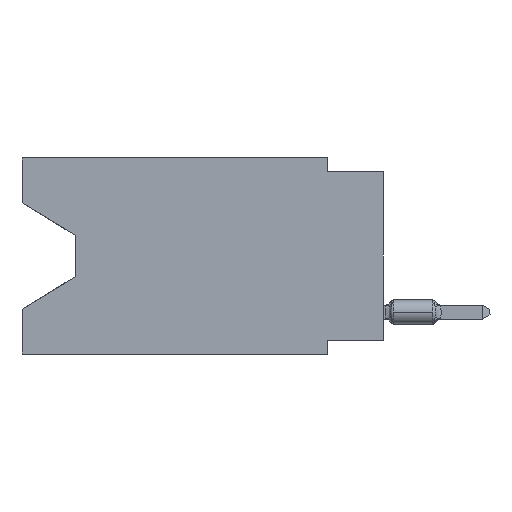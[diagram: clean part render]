
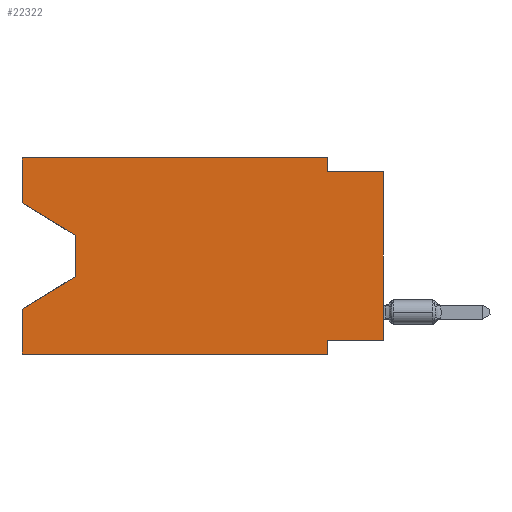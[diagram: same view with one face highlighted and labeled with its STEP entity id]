
A CAD part, left-side view. The second image highlights one B-rep face of the part: STEP entity #22322.
In plain terms, the highlighted planar face has unit normal (-1, 0, 0).
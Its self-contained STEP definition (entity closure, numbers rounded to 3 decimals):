
#72 = CARTESIAN_POINT ( 'NONE',  ( 0., 13.97, -3.505 ) ) ;
#204 = CARTESIAN_POINT ( 'NONE',  ( 0., 16.383, 0. ) ) ;
#387 = EDGE_CURVE ( 'NONE', #8166, #8063, #22553, .T. ) ;
#684 = EDGE_CURVE ( 'NONE', #5565, #3369, #23411, .T. ) ;
#905 = ORIENTED_EDGE ( 'NONE', *, *, #19188, .F. ) ;
#1069 = PLANE ( 'NONE',  #10532 ) ;
#1117 = DIRECTION ( 'NONE',  ( 0., -1., 0. ) ) ;
#1176 = ORIENTED_EDGE ( 'NONE', *, *, #18068, .F. ) ;
#1419 = ORIENTED_EDGE ( 'NONE', *, *, #15341, .T. ) ;
#1423 = VECTOR ( 'NONE', #16731, 1000. ) ;
#1515 = FACE_OUTER_BOUND ( 'NONE', #16196, .T. ) ;
#1603 = VECTOR ( 'NONE', #15028, 1000. ) ;
#1695 = CARTESIAN_POINT ( 'NONE',  ( 0., 16.383, -8.89 ) ) ;
#1734 = CARTESIAN_POINT ( 'NONE',  ( 0., 2.54, 0. ) ) ;
#1870 = ORIENTED_EDGE ( 'NONE', *, *, #10674, .F. ) ;
#1957 = VECTOR ( 'NONE', #16498, 1000. ) ;
#2122 = DIRECTION ( 'NONE',  ( 0., 0., -1. ) ) ;
#2438 = CARTESIAN_POINT ( 'NONE',  ( 0., 0., -0.635 ) ) ;
#2663 = CARTESIAN_POINT ( 'NONE',  ( 0., 16.383, 0. ) ) ;
#2787 = VERTEX_POINT ( 'NONE', #19200 ) ;
#3111 = EDGE_CURVE ( 'NONE', #17561, #3369, #4871, .T. ) ;
#3369 = VERTEX_POINT ( 'NONE', #23626 ) ;
#3672 = LINE ( 'NONE', #1734, #1957 ) ;
#4014 = DIRECTION ( 'NONE',  ( 0., 0., 1. ) ) ;
#4050 = ORIENTED_EDGE ( 'NONE', *, *, #8642, .T. ) ;
#4072 = LINE ( 'NONE', #204, #5555 ) ;
#4871 = LINE ( 'NONE', #19521, #14837 ) ;
#4877 = CARTESIAN_POINT ( 'NONE',  ( 0., 16.383, -8.89 ) ) ;
#4986 = VERTEX_POINT ( 'NONE', #11533 ) ;
#5273 = DIRECTION ( 'NONE',  ( 1., 0., 0. ) ) ;
#5416 = CARTESIAN_POINT ( 'NONE',  ( 0., 13.97, -5.385 ) ) ;
#5555 = VECTOR ( 'NONE', #23937, 1000. ) ;
#5565 = VERTEX_POINT ( 'NONE', #1695 ) ;
#5715 = CARTESIAN_POINT ( 'NONE',  ( 0., 16.383, 0. ) ) ;
#6098 = ORIENTED_EDGE ( 'NONE', *, *, #9938, .F. ) ;
#6109 = EDGE_CURVE ( 'NONE', #5565, #4986, #4072, .T. ) ;
#6717 = VERTEX_POINT ( 'NONE', #11790 ) ;
#6826 = ORIENTED_EDGE ( 'NONE', *, *, #3111, .F. ) ;
#7029 = LINE ( 'NONE', #16697, #22878 ) ;
#8004 = DIRECTION ( 'NONE',  ( 0., -1., 0. ) ) ;
#8063 = VERTEX_POINT ( 'NONE', #21836 ) ;
#8119 = LINE ( 'NONE', #2438, #21179 ) ;
#8166 = VERTEX_POINT ( 'NONE', #16743 ) ;
#8642 = EDGE_CURVE ( 'NONE', #2787, #6717, #15022, .T. ) ;
#8965 = ORIENTED_EDGE ( 'NONE', *, *, #6109, .F. ) ;
#9938 = EDGE_CURVE ( 'NONE', #2787, #17561, #7029, .T. ) ;
#9952 = VERTEX_POINT ( 'NONE', #22154 ) ;
#10509 = VECTOR ( 'NONE', #18791, 1000. ) ;
#10532 = AXIS2_PLACEMENT_3D ( 'NONE', #16412, #5273, #21280 ) ;
#10674 = EDGE_CURVE ( 'NONE', #9952, #17861, #3672, .T. ) ;
#11283 = CARTESIAN_POINT ( 'NONE',  ( 0., 16.383, 0. ) ) ;
#11533 = CARTESIAN_POINT ( 'NONE',  ( 0., 16.383, -6.852 ) ) ;
#11790 = CARTESIAN_POINT ( 'NONE',  ( 0., 0., -0.635 ) ) ;
#11877 = LINE ( 'NONE', #2663, #1603 ) ;
#12407 = VECTOR ( 'NONE', #4014, 1000. ) ;
#12721 = VECTOR ( 'NONE', #1117, 1000. ) ;
#12769 = EDGE_CURVE ( 'NONE', #20177, #4986, #21999, .T. ) ;
#12801 = DIRECTION ( 'NONE',  ( 0., 0.855, -0.519 ) ) ;
#14418 = DIRECTION ( 'NONE',  ( 0., 1., 0. ) ) ;
#14448 = CARTESIAN_POINT ( 'NONE',  ( 0., 2.54, -0.635 ) ) ;
#14547 = VECTOR ( 'NONE', #2122, 1000. ) ;
#14626 = ORIENTED_EDGE ( 'NONE', *, *, #387, .T. ) ;
#14837 = VECTOR ( 'NONE', #19634, 1000. ) ;
#14963 = LINE ( 'NONE', #72, #14547 ) ;
#15022 = LINE ( 'NONE', #16943, #12407 ) ;
#15028 = DIRECTION ( 'NONE',  ( 0., -1., 0. ) ) ;
#15188 = ORIENTED_EDGE ( 'NONE', *, *, #12769, .T. ) ;
#15341 = EDGE_CURVE ( 'NONE', #8063, #20177, #14963, .T. ) ;
#16196 = EDGE_LOOP ( 'NONE', ( #14626, #1419, #15188, #8965, #23176, #6826, #6098, #4050, #905, #1870, #18163, #1176 ) ) ;
#16412 = CARTESIAN_POINT ( 'NONE',  ( 0., 16.383, 0. ) ) ;
#16498 = DIRECTION ( 'NONE',  ( 0., 0., -1. ) ) ;
#16697 = CARTESIAN_POINT ( 'NONE',  ( 0., 0., -8.255 ) ) ;
#16731 = DIRECTION ( 'NONE',  ( 0., 0., 1. ) ) ;
#16743 = CARTESIAN_POINT ( 'NONE',  ( 0., 16.383, -2.038 ) ) ;
#16943 = CARTESIAN_POINT ( 'NONE',  ( 0., 0., 0. ) ) ;
#17561 = VERTEX_POINT ( 'NONE', #22323 ) ;
#17861 = VERTEX_POINT ( 'NONE', #14448 ) ;
#18068 = EDGE_CURVE ( 'NONE', #8166, #21653, #20940, .T. ) ;
#18163 = ORIENTED_EDGE ( 'NONE', *, *, #21790, .F. ) ;
#18650 = VECTOR ( 'NONE', #12801, 1000. ) ;
#18791 = DIRECTION ( 'NONE',  ( 0., -0.855, -0.519 ) ) ;
#19188 = EDGE_CURVE ( 'NONE', #17861, #6717, #8119, .T. ) ;
#19200 = CARTESIAN_POINT ( 'NONE',  ( 0., 0., -8.255 ) ) ;
#19521 = CARTESIAN_POINT ( 'NONE',  ( 0., 2.54, -8.89 ) ) ;
#19634 = DIRECTION ( 'NONE',  ( 0., 0., -1. ) ) ;
#20177 = VERTEX_POINT ( 'NONE', #21467 ) ;
#20268 = CARTESIAN_POINT ( 'NONE',  ( 0., 16.383, -2.038 ) ) ;
#20940 = LINE ( 'NONE', #11283, #1423 ) ;
#21179 = VECTOR ( 'NONE', #8004, 1000. ) ;
#21280 = DIRECTION ( 'NONE',  ( 0., 0., -1. ) ) ;
#21467 = CARTESIAN_POINT ( 'NONE',  ( 0., 13.97, -5.385 ) ) ;
#21653 = VERTEX_POINT ( 'NONE', #5715 ) ;
#21790 = EDGE_CURVE ( 'NONE', #21653, #9952, #11877, .T. ) ;
#21836 = CARTESIAN_POINT ( 'NONE',  ( 0., 13.97, -3.505 ) ) ;
#21999 = LINE ( 'NONE', #5416, #18650 ) ;
#22154 = CARTESIAN_POINT ( 'NONE',  ( 0., 2.54, 0. ) ) ;
#22322 = ADVANCED_FACE ( 'NONE', ( #1515 ), #1069, .F. ) ;
#22323 = CARTESIAN_POINT ( 'NONE',  ( 0., 2.54, -8.255 ) ) ;
#22553 = LINE ( 'NONE', #20268, #10509 ) ;
#22878 = VECTOR ( 'NONE', #14418, 1000. ) ;
#23176 = ORIENTED_EDGE ( 'NONE', *, *, #684, .T. ) ;
#23411 = LINE ( 'NONE', #4877, #12721 ) ;
#23626 = CARTESIAN_POINT ( 'NONE',  ( 0., 2.54, -8.89 ) ) ;
#23937 = DIRECTION ( 'NONE',  ( 0., 0., 1. ) ) ;
